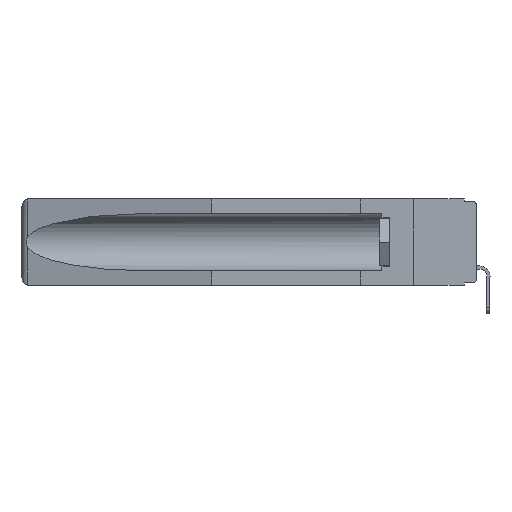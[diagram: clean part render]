
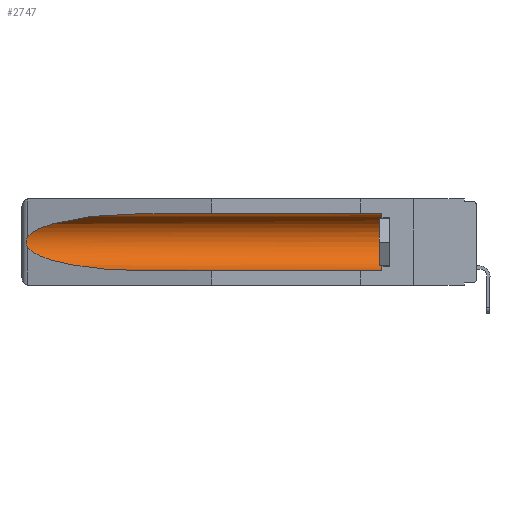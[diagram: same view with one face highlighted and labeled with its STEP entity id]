
A CAD part, left-side view. The second image highlights one B-rep face of the part: STEP entity #2747.
In plain terms, the highlighted cylindrical face has radius 2.857 mm (diameter 5.715 mm), a partial arc.
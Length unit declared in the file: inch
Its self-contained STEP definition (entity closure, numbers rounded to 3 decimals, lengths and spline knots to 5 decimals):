
#286 = CARTESIAN_POINT ( 'NONE',  ( 0.26537, 1.52718, -0.14972 ) ) ;
#870 = CARTESIAN_POINT ( 'NONE',  ( 0.26537, 1.52718, -0.14972 ) ) ;
#1012 = ORIENTED_EDGE ( 'NONE', *, *, #10534, .T. ) ;
#1086 =( BOUNDED_CURVE ( )  B_SPLINE_CURVE ( 3, ( #5201, #13595, #14905, #286 ),
 .UNSPECIFIED., .F., .F. ) 
 B_SPLINE_CURVE_WITH_KNOTS ( ( 4, 4 ),
 ( 4.71239, 6.08839 ),
 .UNSPECIFIED. ) 
 CURVE ( )  GEOMETRIC_REPRESENTATION_ITEM ( )  RATIONAL_B_SPLINE_CURVE ( ( 1., 0.848, 0.848, 1. ) ) 
 REPRESENTATION_ITEM ( '' )  );
#1438 = ORIENTED_EDGE ( 'NONE', *, *, #2692, .T. ) ;
#1548 = AXIS2_PLACEMENT_3D ( 'NONE', #13396, #13450, #3703 ) ;
#1585 = VERTEX_POINT ( 'NONE', #12849 ) ;
#1813 = CARTESIAN_POINT ( 'NONE',  ( 0.2673, 1.5327, -0.16383 ) ) ;
#2507 = FACE_OUTER_BOUND ( 'NONE', #4147, .T. ) ;
#2692 = EDGE_CURVE ( 'NONE', #12092, #15193, #12946, .T. ) ;
#2747 = ADVANCED_FACE ( 'NONE', ( #2507 ), #9509, .F. ) ;
#2998 = ORIENTED_EDGE ( 'NONE', *, *, #7077, .F. ) ;
#3048 = CARTESIAN_POINT ( 'NONE',  ( 0.2675, 1.53308, -0.17534 ) ) ;
#3113 = CARTESIAN_POINT ( 'NONE',  ( 0.155, 0.126, -0.059 ) ) ;
#3503 = EDGE_CURVE ( 'NONE', #15193, #9462, #1086, .T. ) ;
#3703 = DIRECTION ( 'NONE',  ( 0., 0., 1. ) ) ;
#3719 = CARTESIAN_POINT ( 'NONE',  ( 0.155, 1.07973, -0.284 ) ) ;
#3781 = DIRECTION ( 'NONE',  ( 0., 1., 0. ) ) ;
#4147 = EDGE_LOOP ( 'NONE', ( #10572, #1012, #8970, #2998, #15760, #1438 ) ) ;
#4258 = CARTESIAN_POINT ( 'NONE',  ( 0.2673, 1.53269, -0.17917 ) ) ;
#4512 = CARTESIAN_POINT ( 'NONE',  ( 0.21114, 1.30732, -0.284 ) ) ;
#4929 = CARTESIAN_POINT ( 'NONE',  ( 0.155, 1.07973, -0.059 ) ) ;
#5201 = CARTESIAN_POINT ( 'NONE',  ( 0.155, 1.07973, -0.059 ) ) ;
#5475 = CARTESIAN_POINT ( 'NONE',  ( 0.26655, 1.53094, -0.18657 ) ) ;
#6448 = VECTOR ( 'NONE', #3781, 39.37008 ) ;
#6667 = CARTESIAN_POINT ( 'NONE',  ( 0.26537, 1.52718, -0.19328 ) ) ;
#7034 = CARTESIAN_POINT ( 'NONE',  ( 0.26537, 1.52718, -0.19328 ) ) ;
#7077 = EDGE_CURVE ( 'NONE', #1585, #9602, #9141, .T. ) ;
#7316 = DIRECTION ( 'NONE',  ( 0., 1., 0. ) ) ;
#7965 = CARTESIAN_POINT ( 'NONE',  ( 0.155, -0.30754, -0.059 ) ) ;
#8191 = EDGE_CURVE ( 'NONE', #12879, #9602, #15063, .T. ) ;
#8348 = EDGE_CURVE ( 'NONE', #1585, #12092, #11954, .T. ) ;
#8755 = DIRECTION ( 'NONE',  ( 0., 1., 0. ) ) ;
#8970 = ORIENTED_EDGE ( 'NONE', *, *, #8191, .T. ) ;
#8990 = CARTESIAN_POINT ( 'NONE',  ( 0.155, -0.30754, -0.284 ) ) ;
#9141 = LINE ( 'NONE', #8990, #14665 ) ;
#9462 = VERTEX_POINT ( 'NONE', #870 ) ;
#9509 = CYLINDRICAL_SURFACE ( 'NONE', #11270, 0.1125 ) ;
#9602 = VERTEX_POINT ( 'NONE', #12129 ) ;
#10303 = CARTESIAN_POINT ( 'NONE',  ( 0.2675, 1.53308, -0.16763 ) ) ;
#10469 = CARTESIAN_POINT ( 'NONE',  ( 0.155, -0.30754, -0.1715 ) ) ;
#10534 = EDGE_CURVE ( 'NONE', #9462, #12879, #13573, .T. ) ;
#10572 = ORIENTED_EDGE ( 'NONE', *, *, #3503, .T. ) ;
#11270 = AXIS2_PLACEMENT_3D ( 'NONE', #10469, #8755, #13752 ) ;
#11954 = CIRCLE ( 'NONE', #1548, 0.1125 ) ;
#12092 = VERTEX_POINT ( 'NONE', #3113 ) ;
#12129 = CARTESIAN_POINT ( 'NONE',  ( 0.155, 1.07973, -0.284 ) ) ;
#12643 = CARTESIAN_POINT ( 'NONE',  ( 0.26597, 1.52961, -0.15275 ) ) ;
#12758 = CARTESIAN_POINT ( 'NONE',  ( 0.26537, 1.52718, -0.14972 ) ) ;
#12849 = CARTESIAN_POINT ( 'NONE',  ( 0.155, 0.126, -0.284 ) ) ;
#12879 = VERTEX_POINT ( 'NONE', #15756 ) ;
#12946 = LINE ( 'NONE', #7965, #6448 ) ;
#13396 = CARTESIAN_POINT ( 'NONE',  ( 0.155, 0.126, -0.1715 ) ) ;
#13450 = DIRECTION ( 'NONE',  ( 0., -1., 0. ) ) ;
#13573 = B_SPLINE_CURVE_WITH_KNOTS ( 'NONE', 3,
 ( #12758, #12643, #13872, #1813, #10303, #3048, #4258, #5475, #13978, #6667 ),
 .UNSPECIFIED., .F., .F.,
 ( 4, 2, 2, 2, 4 ),
 ( 0., 0.00029, 0.00058, 0.00087, 0.00117 ),
 .UNSPECIFIED. ) ;
#13595 = CARTESIAN_POINT ( 'NONE',  ( 0.21114, 1.30732, -0.059 ) ) ;
#13752 = DIRECTION ( 'NONE',  ( 0., 0., 1. ) ) ;
#13872 = CARTESIAN_POINT ( 'NONE',  ( 0.26654, 1.53092, -0.15636 ) ) ;
#13978 = CARTESIAN_POINT ( 'NONE',  ( 0.26597, 1.5296, -0.19026 ) ) ;
#14245 = CARTESIAN_POINT ( 'NONE',  ( 0.25451, 1.48313, -0.24835 ) ) ;
#14665 = VECTOR ( 'NONE', #7316, 39.37008 ) ;
#14905 = CARTESIAN_POINT ( 'NONE',  ( 0.25451, 1.48313, -0.09465 ) ) ;
#15063 =( BOUNDED_CURVE ( )  B_SPLINE_CURVE ( 3, ( #7034, #14245, #4512, #3719 ),
 .UNSPECIFIED., .F., .F. ) 
 B_SPLINE_CURVE_WITH_KNOTS ( ( 4, 4 ),
 ( 0.1948, 1.5708 ),
 .UNSPECIFIED. ) 
 CURVE ( )  GEOMETRIC_REPRESENTATION_ITEM ( )  RATIONAL_B_SPLINE_CURVE ( ( 1., 0.848, 0.848, 1. ) ) 
 REPRESENTATION_ITEM ( '' )  );
#15193 = VERTEX_POINT ( 'NONE', #4929 ) ;
#15756 = CARTESIAN_POINT ( 'NONE',  ( 0.26537, 1.52718, -0.19328 ) ) ;
#15760 = ORIENTED_EDGE ( 'NONE', *, *, #8348, .T. ) ;
